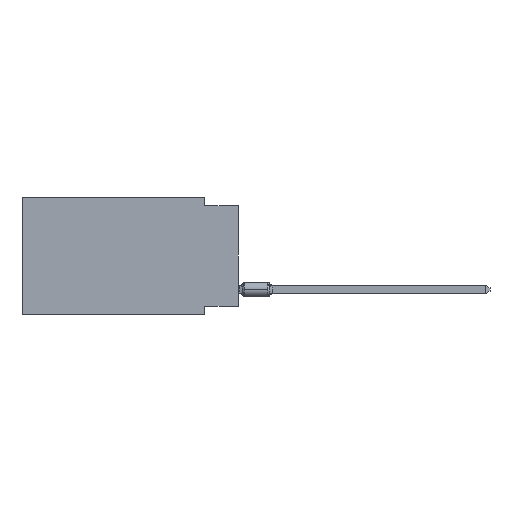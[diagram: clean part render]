
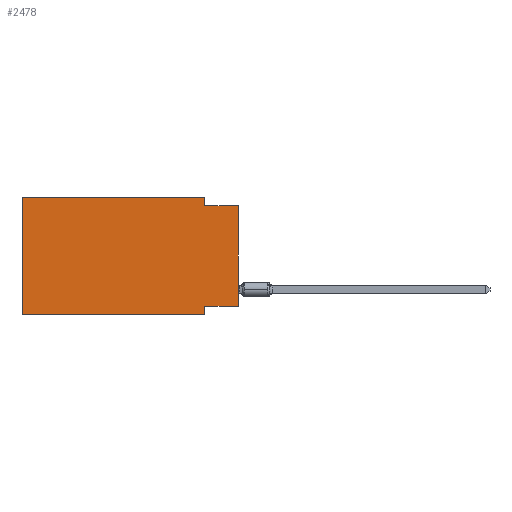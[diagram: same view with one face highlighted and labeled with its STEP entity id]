
A CAD part, left-side view. The second image highlights one B-rep face of the part: STEP entity #2478.
In plain terms, the highlighted planar face has unit normal (-1, 0, 0).
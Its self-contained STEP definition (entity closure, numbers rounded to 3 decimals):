
#323 = ORIENTED_EDGE ( 'NONE', *, *, #12367, .T. ) ;
#478 = CARTESIAN_POINT ( 'NONE',  ( 0., 0., -0.635 ) ) ;
#598 = CARTESIAN_POINT ( 'NONE',  ( 0., 0., 0. ) ) ;
#711 = LINE ( 'NONE', #598, #21799 ) ;
#743 = EDGE_LOOP ( 'NONE', ( #323, #14276, #10835, #11633, #8437, #10536, #1867, #4971 ) ) ;
#1561 = DIRECTION ( 'NONE',  ( 0., 1., 0. ) ) ;
#1867 = ORIENTED_EDGE ( 'NONE', *, *, #1971, .F. ) ;
#1971 = EDGE_CURVE ( 'NONE', #13867, #18600, #2628, .T. ) ;
#2140 = DIRECTION ( 'NONE',  ( 0., 0., 1. ) ) ;
#2478 = ADVANCED_FACE ( 'NONE', ( #14706 ), #20082, .F. ) ;
#2628 = LINE ( 'NONE', #14620, #14218 ) ;
#2750 = VERTEX_POINT ( 'NONE', #3171 ) ;
#2963 = CARTESIAN_POINT ( 'NONE',  ( 0., 0., -8.255 ) ) ;
#3171 = CARTESIAN_POINT ( 'NONE',  ( 0., 16.383, 0. ) ) ;
#3185 = EDGE_CURVE ( 'NONE', #21565, #9477, #22152, .T. ) ;
#3198 = LINE ( 'NONE', #19182, #14996 ) ;
#3829 = LINE ( 'NONE', #478, #18440 ) ;
#4854 = CARTESIAN_POINT ( 'NONE',  ( 0., 0., -8.255 ) ) ;
#4971 = ORIENTED_EDGE ( 'NONE', *, *, #18097, .F. ) ;
#5468 = LINE ( 'NONE', #16304, #16265 ) ;
#6010 = DIRECTION ( 'NONE',  ( 0., 0., 1. ) ) ;
#6245 = CARTESIAN_POINT ( 'NONE',  ( 0., 2.54, 0. ) ) ;
#6742 = CARTESIAN_POINT ( 'NONE',  ( 0., 2.54, -0.635 ) ) ;
#7841 = CARTESIAN_POINT ( 'NONE',  ( 0., 2.54, -8.255 ) ) ;
#8437 = ORIENTED_EDGE ( 'NONE', *, *, #9647, .F. ) ;
#9477 = VERTEX_POINT ( 'NONE', #6742 ) ;
#9647 = EDGE_CURVE ( 'NONE', #19696, #2750, #5468, .T. ) ;
#10096 = EDGE_CURVE ( 'NONE', #9477, #12731, #3829, .T. ) ;
#10358 = EDGE_CURVE ( 'NONE', #2750, #21565, #22433, .T. ) ;
#10536 = ORIENTED_EDGE ( 'NONE', *, *, #15502, .T. ) ;
#10795 = DIRECTION ( 'NONE',  ( 1., 0., 0. ) ) ;
#10835 = ORIENTED_EDGE ( 'NONE', *, *, #3185, .F. ) ;
#10918 = AXIS2_PLACEMENT_3D ( 'NONE', #19750, #10795, #16553 ) ;
#11633 = ORIENTED_EDGE ( 'NONE', *, *, #10358, .F. ) ;
#11834 = LINE ( 'NONE', #2963, #15415 ) ;
#11994 = CARTESIAN_POINT ( 'NONE',  ( 0., 16.383, 0. ) ) ;
#12367 = EDGE_CURVE ( 'NONE', #18351, #12731, #711, .T. ) ;
#12731 = VERTEX_POINT ( 'NONE', #22422 ) ;
#13691 = CARTESIAN_POINT ( 'NONE',  ( 0., 2.54, 0. ) ) ;
#13867 = VERTEX_POINT ( 'NONE', #7841 ) ;
#14218 = VECTOR ( 'NONE', #19664, 1000. ) ;
#14276 = ORIENTED_EDGE ( 'NONE', *, *, #10096, .F. ) ;
#14620 = CARTESIAN_POINT ( 'NONE',  ( 0., 2.54, -8.89 ) ) ;
#14706 = FACE_OUTER_BOUND ( 'NONE', #743, .T. ) ;
#14996 = VECTOR ( 'NONE', #17256, 1000. ) ;
#15415 = VECTOR ( 'NONE', #1561, 1000. ) ;
#15502 = EDGE_CURVE ( 'NONE', #19696, #18600, #3198, .T. ) ;
#16265 = VECTOR ( 'NONE', #2140, 1000. ) ;
#16304 = CARTESIAN_POINT ( 'NONE',  ( 0., 16.383, 0. ) ) ;
#16472 = VECTOR ( 'NONE', #20317, 1000. ) ;
#16553 = DIRECTION ( 'NONE',  ( 0., 0., -1. ) ) ;
#17256 = DIRECTION ( 'NONE',  ( 0., -1., 0. ) ) ;
#18097 = EDGE_CURVE ( 'NONE', #18351, #13867, #11834, .T. ) ;
#18351 = VERTEX_POINT ( 'NONE', #4854 ) ;
#18440 = VECTOR ( 'NONE', #21524, 1000. ) ;
#18600 = VERTEX_POINT ( 'NONE', #19897 ) ;
#18885 = DIRECTION ( 'NONE',  ( 0., -1., 0. ) ) ;
#19182 = CARTESIAN_POINT ( 'NONE',  ( 0., 16.383, -8.89 ) ) ;
#19664 = DIRECTION ( 'NONE',  ( 0., 0., -1. ) ) ;
#19696 = VERTEX_POINT ( 'NONE', #20633 ) ;
#19750 = CARTESIAN_POINT ( 'NONE',  ( 0., 16.383, 0. ) ) ;
#19897 = CARTESIAN_POINT ( 'NONE',  ( 0., 2.54, -8.89 ) ) ;
#20082 = PLANE ( 'NONE',  #10918 ) ;
#20317 = DIRECTION ( 'NONE',  ( 0., 0., -1. ) ) ;
#20633 = CARTESIAN_POINT ( 'NONE',  ( 0., 16.383, -8.89 ) ) ;
#21524 = DIRECTION ( 'NONE',  ( 0., -1., 0. ) ) ;
#21565 = VERTEX_POINT ( 'NONE', #6245 ) ;
#21799 = VECTOR ( 'NONE', #6010, 1000. ) ;
#22114 = VECTOR ( 'NONE', #18885, 1000. ) ;
#22152 = LINE ( 'NONE', #13691, #16472 ) ;
#22422 = CARTESIAN_POINT ( 'NONE',  ( 0., 0., -0.635 ) ) ;
#22433 = LINE ( 'NONE', #11994, #22114 ) ;
